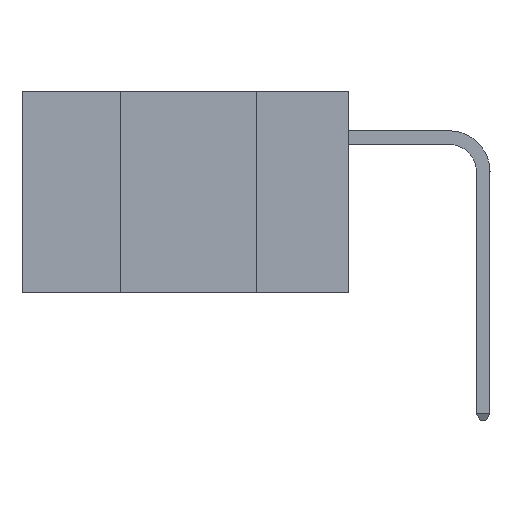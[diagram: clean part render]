
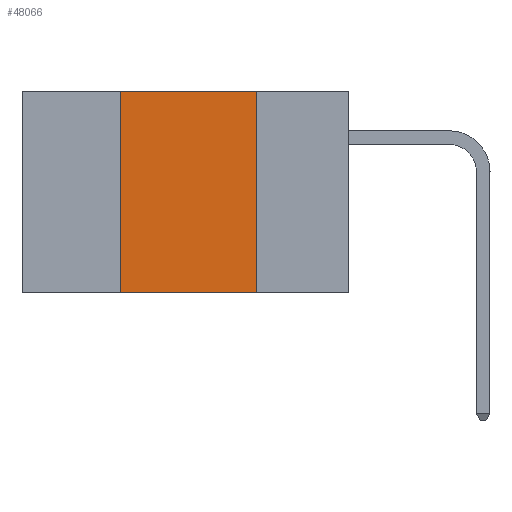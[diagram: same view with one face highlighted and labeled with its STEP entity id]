
A CAD part, left-side view. The second image highlights one B-rep face of the part: STEP entity #48066.
In plain terms, the highlighted planar face has unit normal (-1, 0, 0).
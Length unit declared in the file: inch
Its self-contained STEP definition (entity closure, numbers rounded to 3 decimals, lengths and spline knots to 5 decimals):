
#504 = FACE_OUTER_BOUND ( 'NONE', #5572, .T. ) ;
#2968 = CARTESIAN_POINT ( 'NONE',  ( 0., 0.42, 0. ) ) ;
#3844 = EDGE_CURVE ( 'NONE', #38480, #44997, #5365, .T. ) ;
#4185 = VECTOR ( 'NONE', #35947, 39.37008 ) ;
#5000 = EDGE_CURVE ( 'NONE', #44997, #14621, #17898, .T. ) ;
#5365 = LINE ( 'NONE', #9140, #4185 ) ;
#5572 = EDGE_LOOP ( 'NONE', ( #26460, #32255, #20304, #14823 ) ) ;
#6726 = PLANE ( 'NONE',  #27941 ) ;
#7675 = VECTOR ( 'NONE', #33794, 39.37008 ) ;
#8712 = DIRECTION ( 'NONE',  ( 0., -1., 0. ) ) ;
#9140 = CARTESIAN_POINT ( 'NONE',  ( 0., 0.6, 0. ) ) ;
#10615 = DIRECTION ( 'NONE',  ( 1., 0., 0. ) ) ;
#13454 = EDGE_CURVE ( 'NONE', #48400, #14621, #16739, .T. ) ;
#14621 = VERTEX_POINT ( 'NONE', #31424 ) ;
#14823 = ORIENTED_EDGE ( 'NONE', *, *, #13454, .T. ) ;
#16739 = LINE ( 'NONE', #31676, #37074 ) ;
#17898 = LINE ( 'NONE', #26174, #7675 ) ;
#20304 = ORIENTED_EDGE ( 'NONE', *, *, #27950, .F. ) ;
#22048 = CARTESIAN_POINT ( 'NONE',  ( 0., 0.6, 0. ) ) ;
#26174 = CARTESIAN_POINT ( 'NONE',  ( 0., 0.17, 0. ) ) ;
#26460 = ORIENTED_EDGE ( 'NONE', *, *, #5000, .F. ) ;
#27941 = AXIS2_PLACEMENT_3D ( 'NONE', #22048, #10615, #37401 ) ;
#27950 = EDGE_CURVE ( 'NONE', #48400, #38480, #33496, .T. ) ;
#31344 = CARTESIAN_POINT ( 'NONE',  ( 0., 0.42, 0. ) ) ;
#31424 = CARTESIAN_POINT ( 'NONE',  ( 0., 0.17, -0.37 ) ) ;
#31676 = CARTESIAN_POINT ( 'NONE',  ( 0., 0.6, -0.37 ) ) ;
#32255 = ORIENTED_EDGE ( 'NONE', *, *, #3844, .F. ) ;
#33496 = LINE ( 'NONE', #2968, #42498 ) ;
#33621 = DIRECTION ( 'NONE',  ( 0., 0., 1. ) ) ;
#33794 = DIRECTION ( 'NONE',  ( 0., 0., -1. ) ) ;
#35947 = DIRECTION ( 'NONE',  ( 0., -1., 0. ) ) ;
#37074 = VECTOR ( 'NONE', #8712, 39.37008 ) ;
#37401 = DIRECTION ( 'NONE',  ( 0., 0., -1. ) ) ;
#38480 = VERTEX_POINT ( 'NONE', #31344 ) ;
#42498 = VECTOR ( 'NONE', #33621, 39.37008 ) ;
#43592 = CARTESIAN_POINT ( 'NONE',  ( 0., 0.42, -0.37 ) ) ;
#44138 = CARTESIAN_POINT ( 'NONE',  ( 0., 0.17, 0. ) ) ;
#44997 = VERTEX_POINT ( 'NONE', #44138 ) ;
#48066 = ADVANCED_FACE ( 'NONE', ( #504 ), #6726, .F. ) ;
#48400 = VERTEX_POINT ( 'NONE', #43592 ) ;
